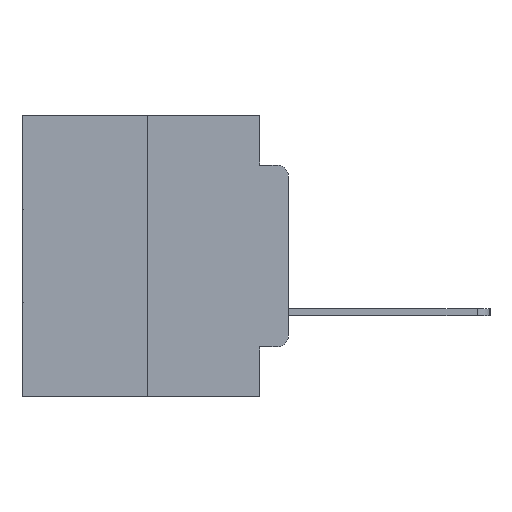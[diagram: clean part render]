
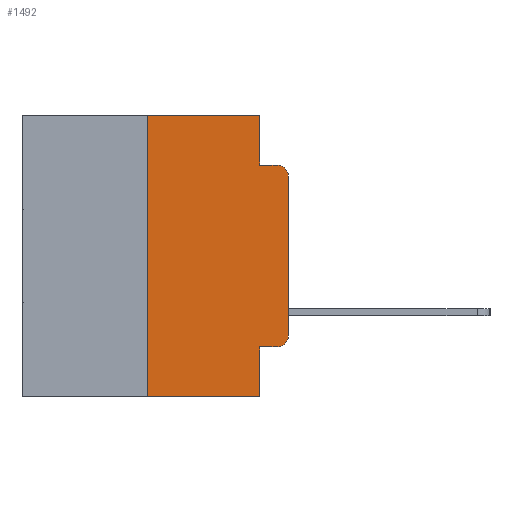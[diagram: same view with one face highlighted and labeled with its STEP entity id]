
A CAD part, left-side view. The second image highlights one B-rep face of the part: STEP entity #1492.
In plain terms, the highlighted planar face has unit normal (-1, 0, 0).
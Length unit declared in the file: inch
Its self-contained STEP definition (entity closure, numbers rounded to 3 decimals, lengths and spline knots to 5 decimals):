
#160 = DIRECTION ( 'NONE',  ( 0., -1., 0. ) ) ;
#1165 = VERTEX_POINT ( 'NONE', #12578 ) ;
#1448 = ORIENTED_EDGE ( 'NONE', *, *, #6062, .T. ) ;
#1492 = ADVANCED_FACE ( 'NONE', ( #5421 ), #2241, .F. ) ;
#2241 = PLANE ( 'NONE',  #11957 ) ;
#2562 = LINE ( 'NONE', #27519, #20103 ) ;
#3379 = VECTOR ( 'NONE', #13769, 39.37008 ) ;
#3505 = DIRECTION ( 'NONE',  ( -1., 0., 0. ) ) ;
#3813 = DIRECTION ( 'NONE',  ( -1., 0., 0. ) ) ;
#4507 = CARTESIAN_POINT ( 'NONE',  ( 0., 0., -0.3915 ) ) ;
#4538 = EDGE_CURVE ( 'NONE', #23043, #19519, #9555, .T. ) ;
#4546 = DIRECTION ( 'NONE',  ( 0., 0., -1. ) ) ;
#4918 = DIRECTION ( 'NONE',  ( 0., -1., 0. ) ) ;
#4993 = CARTESIAN_POINT ( 'NONE',  ( 0., 0., 0. ) ) ;
#5421 = FACE_OUTER_BOUND ( 'NONE', #25758, .T. ) ;
#5658 = DIRECTION ( 'NONE',  ( 0., -1., 0. ) ) ;
#5733 = DIRECTION ( 'NONE',  ( 0., 0., -1. ) ) ;
#6062 = EDGE_CURVE ( 'NONE', #7077, #23043, #21281, .T. ) ;
#6985 = LINE ( 'NONE', #11987, #18474 ) ;
#7077 = VERTEX_POINT ( 'NONE', #21057 ) ;
#7132 = ORIENTED_EDGE ( 'NONE', *, *, #21426, .T. ) ;
#7182 = VECTOR ( 'NONE', #25634, 39.37008 ) ;
#7246 = DIRECTION ( 'NONE',  ( 0., 0., 1. ) ) ;
#7610 = EDGE_CURVE ( 'NONE', #19018, #7983, #2562, .T. ) ;
#7983 = VERTEX_POINT ( 'NONE', #15185 ) ;
#8843 = CARTESIAN_POINT ( 'NONE',  ( 0., 0., -0.1085 ) ) ;
#9555 = CIRCLE ( 'NONE', #21590, 0.02 ) ;
#9841 = ORIENTED_EDGE ( 'NONE', *, *, #19709, .T. ) ;
#10247 = CARTESIAN_POINT ( 'NONE',  ( 0., 0.051, -0.0885 ) ) ;
#10524 = VECTOR ( 'NONE', #4918, 39.37008 ) ;
#11471 = CARTESIAN_POINT ( 'NONE',  ( 0., 0.051, 0. ) ) ;
#11941 = LINE ( 'NONE', #4993, #23388 ) ;
#11957 = AXIS2_PLACEMENT_3D ( 'NONE', #15953, #18255, #4546 ) ;
#11987 = CARTESIAN_POINT ( 'NONE',  ( 0., 0.473, -0.5 ) ) ;
#12175 = VERTEX_POINT ( 'NONE', #8843 ) ;
#12223 = CARTESIAN_POINT ( 'NONE',  ( 0., 0.02, -0.0885 ) ) ;
#12237 = EDGE_CURVE ( 'NONE', #7077, #22922, #21649, .T. ) ;
#12578 = CARTESIAN_POINT ( 'NONE',  ( 0., 0.051, -0.0885 ) ) ;
#13457 = LINE ( 'NONE', #10247, #25560 ) ;
#13754 = EDGE_CURVE ( 'NONE', #26360, #19018, #17963, .T. ) ;
#13769 = DIRECTION ( 'NONE',  ( 0., 0., -1. ) ) ;
#14286 = DIRECTION ( 'NONE',  ( 0., -1., 0. ) ) ;
#15066 = ORIENTED_EDGE ( 'NONE', *, *, #19887, .F. ) ;
#15185 = CARTESIAN_POINT ( 'NONE',  ( 0., 0.051, 0. ) ) ;
#15288 = EDGE_CURVE ( 'NONE', #7983, #1165, #21571, .T. ) ;
#15953 = CARTESIAN_POINT ( 'NONE',  ( 0., 0.473, 0. ) ) ;
#16336 = VERTEX_POINT ( 'NONE', #12223 ) ;
#16460 = CARTESIAN_POINT ( 'NONE',  ( 0., 0.25, 0. ) ) ;
#16573 = CARTESIAN_POINT ( 'NONE',  ( 0., 0.25, -0.5 ) ) ;
#17203 = CARTESIAN_POINT ( 'NONE',  ( 0., 0.02, -0.3915 ) ) ;
#17512 = CARTESIAN_POINT ( 'NONE',  ( 0., 0.02, -0.1085 ) ) ;
#17963 = LINE ( 'NONE', #23404, #7182 ) ;
#18255 = DIRECTION ( 'NONE',  ( 1., 0., 0. ) ) ;
#18406 = ORIENTED_EDGE ( 'NONE', *, *, #13754, .F. ) ;
#18474 = VECTOR ( 'NONE', #14286, 39.37008 ) ;
#18645 = CARTESIAN_POINT ( 'NONE',  ( 0., 0.051, -0.4115 ) ) ;
#19018 = VERTEX_POINT ( 'NONE', #16460 ) ;
#19081 = ORIENTED_EDGE ( 'NONE', *, *, #15288, .F. ) ;
#19306 = ORIENTED_EDGE ( 'NONE', *, *, #12237, .F. ) ;
#19510 = DIRECTION ( 'NONE',  ( 0., 0., -1. ) ) ;
#19519 = VERTEX_POINT ( 'NONE', #4507 ) ;
#19690 = ORIENTED_EDGE ( 'NONE', *, *, #22947, .T. ) ;
#19709 = EDGE_CURVE ( 'NONE', #26360, #22922, #6985, .T. ) ;
#19815 = DIRECTION ( 'NONE',  ( 0., 0., -1. ) ) ;
#19887 = EDGE_CURVE ( 'NONE', #1165, #16336, #13457, .T. ) ;
#20103 = VECTOR ( 'NONE', #160, 39.37008 ) ;
#20870 = VECTOR ( 'NONE', #5733, 39.37008 ) ;
#21057 = CARTESIAN_POINT ( 'NONE',  ( 0., 0.051, -0.4115 ) ) ;
#21281 = LINE ( 'NONE', #18645, #10524 ) ;
#21426 = EDGE_CURVE ( 'NONE', #12175, #16336, #28383, .T. ) ;
#21571 = LINE ( 'NONE', #26180, #20870 ) ;
#21590 = AXIS2_PLACEMENT_3D ( 'NONE', #17203, #3505, #19510 ) ;
#21649 = LINE ( 'NONE', #11471, #3379 ) ;
#22922 = VERTEX_POINT ( 'NONE', #27606 ) ;
#22947 = EDGE_CURVE ( 'NONE', #19519, #12175, #11941, .T. ) ;
#23043 = VERTEX_POINT ( 'NONE', #28093 ) ;
#23388 = VECTOR ( 'NONE', #7246, 39.37008 ) ;
#23404 = CARTESIAN_POINT ( 'NONE',  ( 0., 0.25, 0. ) ) ;
#23650 = AXIS2_PLACEMENT_3D ( 'NONE', #17512, #3813, #19815 ) ;
#25560 = VECTOR ( 'NONE', #5658, 39.37008 ) ;
#25634 = DIRECTION ( 'NONE',  ( 0., 0., 1. ) ) ;
#25758 = EDGE_LOOP ( 'NONE', ( #19690, #7132, #15066, #19081, #28595, #18406, #9841, #19306, #1448, #26806 ) ) ;
#26180 = CARTESIAN_POINT ( 'NONE',  ( 0., 0.051, 0. ) ) ;
#26360 = VERTEX_POINT ( 'NONE', #16573 ) ;
#26806 = ORIENTED_EDGE ( 'NONE', *, *, #4538, .T. ) ;
#27519 = CARTESIAN_POINT ( 'NONE',  ( 0., 0.473, 0. ) ) ;
#27606 = CARTESIAN_POINT ( 'NONE',  ( 0., 0.051, -0.5 ) ) ;
#28093 = CARTESIAN_POINT ( 'NONE',  ( 0., 0.02, -0.4115 ) ) ;
#28383 = CIRCLE ( 'NONE', #23650, 0.02 ) ;
#28595 = ORIENTED_EDGE ( 'NONE', *, *, #7610, .F. ) ;
